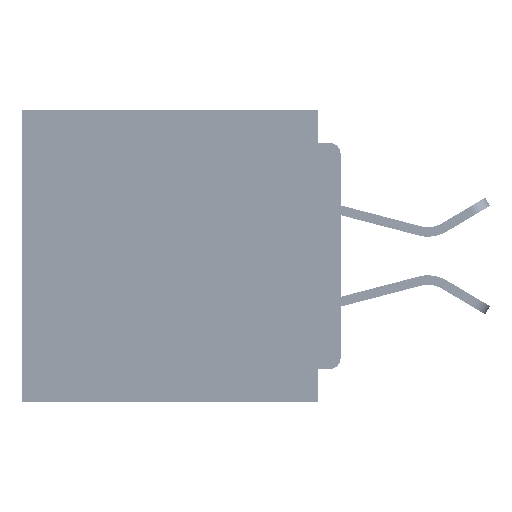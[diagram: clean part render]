
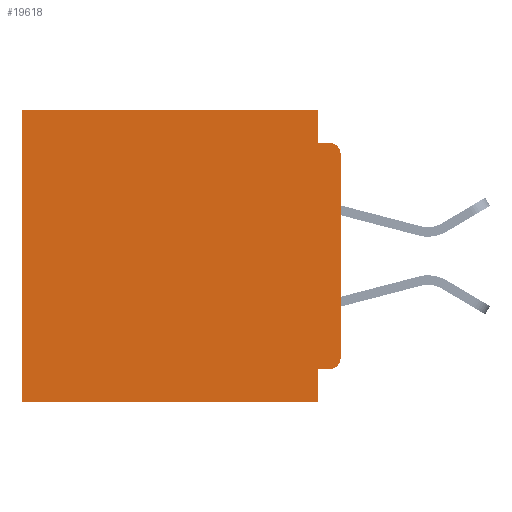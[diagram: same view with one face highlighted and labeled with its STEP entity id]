
A CAD part, left-side view. The second image highlights one B-rep face of the part: STEP entity #19618.
In plain terms, the highlighted planar face has unit normal (-1, 0, 0).
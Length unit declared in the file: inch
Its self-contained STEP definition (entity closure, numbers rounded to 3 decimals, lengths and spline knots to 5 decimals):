
#323 = DIRECTION ( 'NONE',  ( 0., 1., 0. ) ) ;
#334 = EDGE_CURVE ( 'NONE', #60360, #17848, #55755, .T. ) ;
#821 = EDGE_CURVE ( 'NONE', #57210, #33292, #14789, .T. ) ;
#972 = LINE ( 'NONE', #57081, #37288 ) ;
#1650 = VECTOR ( 'NONE', #26479, 39.37008 ) ;
#2451 = CARTESIAN_POINT ( 'NONE',  ( 0.3, 0.437, -0.4 ) ) ;
#6530 = CARTESIAN_POINT ( 'NONE',  ( 0.3, 0.437, -0.4 ) ) ;
#6767 = DIRECTION ( 'NONE',  ( 1., 0., 0. ) ) ;
#9083 = CARTESIAN_POINT ( 'NONE',  ( 0.3, 0., -0.4 ) ) ;
#11476 = CIRCLE ( 'NONE', #54409, 0.015 ) ;
#12900 = LINE ( 'NONE', #23437, #37619 ) ;
#13080 = VECTOR ( 'NONE', #36999, 39.37008 ) ;
#13241 = CARTESIAN_POINT ( 'NONE',  ( 0.3, 0.031, -0.355 ) ) ;
#13310 = VERTEX_POINT ( 'NONE', #14937 ) ;
#13588 = DIRECTION ( 'NONE',  ( -1., 0., 0. ) ) ;
#14072 = DIRECTION ( 'NONE',  ( 0., 0., -1. ) ) ;
#14789 = LINE ( 'NONE', #20099, #1650 ) ;
#14937 = CARTESIAN_POINT ( 'NONE',  ( 0.3, 0.031, 0. ) ) ;
#16482 = CARTESIAN_POINT ( 'NONE',  ( 0.3, 0., -0.4 ) ) ;
#16741 = ORIENTED_EDGE ( 'NONE', *, *, #40231, .T. ) ;
#17848 = VERTEX_POINT ( 'NONE', #31357 ) ;
#19618 = ADVANCED_FACE ( 'NONE', ( #60472 ), #36338, .F. ) ;
#20099 = CARTESIAN_POINT ( 'NONE',  ( 0.3, 0., -0.045 ) ) ;
#20350 = LINE ( 'NONE', #2451, #13080 ) ;
#23437 = CARTESIAN_POINT ( 'NONE',  ( 0.3, 0., -0.355 ) ) ;
#24313 = DIRECTION ( 'NONE',  ( -1., 0., 0. ) ) ;
#26479 = DIRECTION ( 'NONE',  ( 0., -1., 0. ) ) ;
#26776 = ORIENTED_EDGE ( 'NONE', *, *, #36556, .F. ) ;
#27555 = EDGE_CURVE ( 'NONE', #35983, #51440, #11476, .T. ) ;
#27805 = AXIS2_PLACEMENT_3D ( 'NONE', #53856, #24313, #58809 ) ;
#30386 = VECTOR ( 'NONE', #53724, 39.37008 ) ;
#31357 = CARTESIAN_POINT ( 'NONE',  ( 0.3, 0.031, -0.4 ) ) ;
#31579 = CARTESIAN_POINT ( 'NONE',  ( 0.3, 0.437, 0. ) ) ;
#31592 = ORIENTED_EDGE ( 'NONE', *, *, #43456, .F. ) ;
#32026 = CARTESIAN_POINT ( 'NONE',  ( 0.3, 0.015, -0.045 ) ) ;
#32697 = CARTESIAN_POINT ( 'NONE',  ( 0.3, 0.031, -0.4 ) ) ;
#33136 = DIRECTION ( 'NONE',  ( 0., 1., 0. ) ) ;
#33292 = VERTEX_POINT ( 'NONE', #32026 ) ;
#33632 = CARTESIAN_POINT ( 'NONE',  ( 0.3, 0.031, -0.045 ) ) ;
#33900 = CARTESIAN_POINT ( 'NONE',  ( 0.3, 0.031, 0. ) ) ;
#34775 = EDGE_CURVE ( 'NONE', #35983, #60360, #12900, .T. ) ;
#35983 = VERTEX_POINT ( 'NONE', #44546 ) ;
#36338 = PLANE ( 'NONE',  #39181 ) ;
#36556 = EDGE_CURVE ( 'NONE', #13310, #57210, #43511, .T. ) ;
#36999 = DIRECTION ( 'NONE',  ( 0., 0., -1. ) ) ;
#37288 = VECTOR ( 'NONE', #42232, 39.37008 ) ;
#37619 = VECTOR ( 'NONE', #33136, 39.37008 ) ;
#37695 = VECTOR ( 'NONE', #323, 39.37008 ) ;
#38225 = VECTOR ( 'NONE', #14072, 39.37008 ) ;
#38667 = EDGE_CURVE ( 'NONE', #54668, #44758, #20350, .T. ) ;
#39181 = AXIS2_PLACEMENT_3D ( 'NONE', #16482, #6767, #41299 ) ;
#40231 = EDGE_CURVE ( 'NONE', #13310, #54668, #50841, .T. ) ;
#41057 = DIRECTION ( 'NONE',  ( 0., 0., -1. ) ) ;
#41299 = DIRECTION ( 'NONE',  ( 0., 0., -1. ) ) ;
#42232 = DIRECTION ( 'NONE',  ( 0., 1., 0. ) ) ;
#42657 = VECTOR ( 'NONE', #41057, 39.37008 ) ;
#43178 = CARTESIAN_POINT ( 'NONE',  ( 0.3, 0.015, -0.34 ) ) ;
#43456 = EDGE_CURVE ( 'NONE', #17848, #44758, #972, .T. ) ;
#43511 = LINE ( 'NONE', #33900, #30386 ) ;
#44546 = CARTESIAN_POINT ( 'NONE',  ( 0.3, 0.015, -0.355 ) ) ;
#44758 = VERTEX_POINT ( 'NONE', #6530 ) ;
#44821 = CARTESIAN_POINT ( 'NONE',  ( 0.3, 0., 0. ) ) ;
#46087 = ORIENTED_EDGE ( 'NONE', *, *, #38667, .T. ) ;
#47631 = CARTESIAN_POINT ( 'NONE',  ( 0.3, 0., -0.34 ) ) ;
#48144 = DIRECTION ( 'NONE',  ( 0., 0., -1. ) ) ;
#50453 = EDGE_CURVE ( 'NONE', #62043, #51440, #51381, .T. ) ;
#50841 = LINE ( 'NONE', #44821, #37695 ) ;
#51330 = CIRCLE ( 'NONE', #27805, 0.015 ) ;
#51381 = LINE ( 'NONE', #9083, #38225 ) ;
#51440 = VERTEX_POINT ( 'NONE', #47631 ) ;
#51593 = EDGE_CURVE ( 'NONE', #62043, #33292, #51330, .T. ) ;
#53724 = DIRECTION ( 'NONE',  ( 0., 0., -1. ) ) ;
#53856 = CARTESIAN_POINT ( 'NONE',  ( 0.3, 0.015, -0.06 ) ) ;
#54318 = ORIENTED_EDGE ( 'NONE', *, *, #50453, .F. ) ;
#54409 = AXIS2_PLACEMENT_3D ( 'NONE', #43178, #13588, #48144 ) ;
#54429 = ORIENTED_EDGE ( 'NONE', *, *, #51593, .T. ) ;
#54668 = VERTEX_POINT ( 'NONE', #31579 ) ;
#55755 = LINE ( 'NONE', #32697, #42657 ) ;
#57081 = CARTESIAN_POINT ( 'NONE',  ( 0.3, 0., -0.4 ) ) ;
#57210 = VERTEX_POINT ( 'NONE', #33632 ) ;
#58809 = DIRECTION ( 'NONE',  ( 0., 0., -1. ) ) ;
#59129 = CARTESIAN_POINT ( 'NONE',  ( 0.3, 0., -0.06 ) ) ;
#59727 = EDGE_LOOP ( 'NONE', ( #54318, #54429, #62151, #26776, #16741, #46087, #31592, #62870, #62589, #60817 ) ) ;
#60360 = VERTEX_POINT ( 'NONE', #13241 ) ;
#60472 = FACE_OUTER_BOUND ( 'NONE', #59727, .T. ) ;
#60817 = ORIENTED_EDGE ( 'NONE', *, *, #27555, .T. ) ;
#62043 = VERTEX_POINT ( 'NONE', #59129 ) ;
#62151 = ORIENTED_EDGE ( 'NONE', *, *, #821, .F. ) ;
#62589 = ORIENTED_EDGE ( 'NONE', *, *, #34775, .F. ) ;
#62870 = ORIENTED_EDGE ( 'NONE', *, *, #334, .F. ) ;
